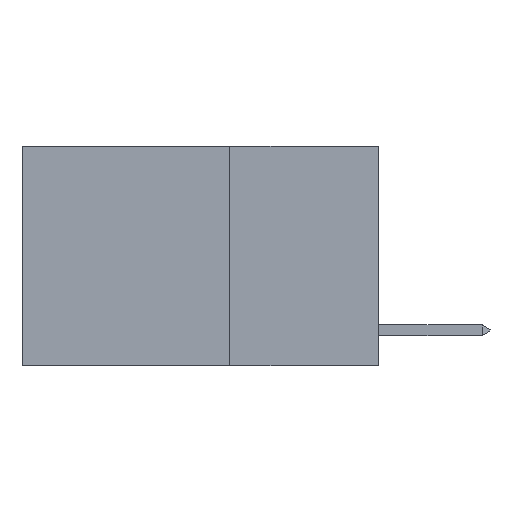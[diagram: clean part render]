
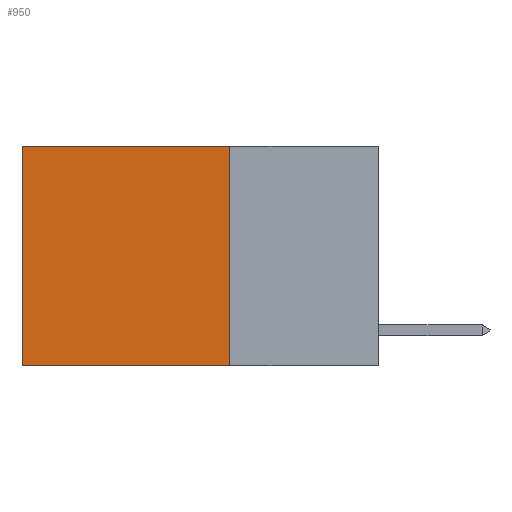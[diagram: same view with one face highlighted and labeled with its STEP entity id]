
A CAD part, left-side view. The second image highlights one B-rep face of the part: STEP entity #950.
In plain terms, the highlighted planar face has unit normal (-1, 0, 0).
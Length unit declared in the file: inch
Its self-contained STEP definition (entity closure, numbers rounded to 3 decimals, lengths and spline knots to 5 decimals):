
#425 = DIRECTION ( 'NONE',  ( 0., 1., 0. ) ) ;
#942 = ORIENTED_EDGE ( 'NONE', *, *, #18204, .T. ) ;
#950 = ADVANCED_FACE ( 'NONE', ( #16349 ), #19726, .F. ) ;
#1105 = CARTESIAN_POINT ( 'NONE',  ( 0.2625, 0.6, 0. ) ) ;
#1932 = VECTOR ( 'NONE', #14367, 39.37008 ) ;
#1953 = LINE ( 'NONE', #8195, #11697 ) ;
#4800 = EDGE_LOOP ( 'NONE', ( #942, #21335, #19915, #15224 ) ) ;
#4982 = VECTOR ( 'NONE', #425, 39.37008 ) ;
#7093 = CARTESIAN_POINT ( 'NONE',  ( 0.2625, 0.25, 0. ) ) ;
#7301 = AXIS2_PLACEMENT_3D ( 'NONE', #7093, #24023, #13387 ) ;
#8195 = CARTESIAN_POINT ( 'NONE',  ( 0.2625, 0.6, 0. ) ) ;
#8366 = CARTESIAN_POINT ( 'NONE',  ( 0.2625, 0.25, -0.37 ) ) ;
#8734 = VERTEX_POINT ( 'NONE', #19347 ) ;
#9211 = VECTOR ( 'NONE', #23041, 39.37008 ) ;
#9443 = EDGE_CURVE ( 'NONE', #14467, #8734, #20081, .T. ) ;
#10579 = CARTESIAN_POINT ( 'NONE',  ( 0.2625, 0.25, 0. ) ) ;
#11697 = VECTOR ( 'NONE', #21301, 39.37008 ) ;
#12171 = CARTESIAN_POINT ( 'NONE',  ( 0.2625, 0.25, -0.37 ) ) ;
#13387 = DIRECTION ( 'NONE',  ( 0., 0., -1. ) ) ;
#13594 = VERTEX_POINT ( 'NONE', #23887 ) ;
#14367 = DIRECTION ( 'NONE',  ( 0., 1., 0. ) ) ;
#14467 = VERTEX_POINT ( 'NONE', #8366 ) ;
#14812 = LINE ( 'NONE', #21221, #9211 ) ;
#15224 = ORIENTED_EDGE ( 'NONE', *, *, #19275, .T. ) ;
#16349 = FACE_OUTER_BOUND ( 'NONE', #4800, .T. ) ;
#17299 = LINE ( 'NONE', #10579, #1932 ) ;
#18204 = EDGE_CURVE ( 'NONE', #21728, #8734, #1953, .T. ) ;
#19275 = EDGE_CURVE ( 'NONE', #13594, #21728, #17299, .T. ) ;
#19347 = CARTESIAN_POINT ( 'NONE',  ( 0.2625, 0.6, -0.37 ) ) ;
#19726 = PLANE ( 'NONE',  #7301 ) ;
#19915 = ORIENTED_EDGE ( 'NONE', *, *, #22372, .F. ) ;
#20081 = LINE ( 'NONE', #12171, #4982 ) ;
#21221 = CARTESIAN_POINT ( 'NONE',  ( 0.2625, 0.25, 0. ) ) ;
#21301 = DIRECTION ( 'NONE',  ( 0., 0., -1. ) ) ;
#21335 = ORIENTED_EDGE ( 'NONE', *, *, #9443, .F. ) ;
#21728 = VERTEX_POINT ( 'NONE', #1105 ) ;
#22372 = EDGE_CURVE ( 'NONE', #13594, #14467, #14812, .T. ) ;
#23041 = DIRECTION ( 'NONE',  ( 0., 0., -1. ) ) ;
#23887 = CARTESIAN_POINT ( 'NONE',  ( 0.2625, 0.25, 0. ) ) ;
#24023 = DIRECTION ( 'NONE',  ( 1., 0., 0. ) ) ;
